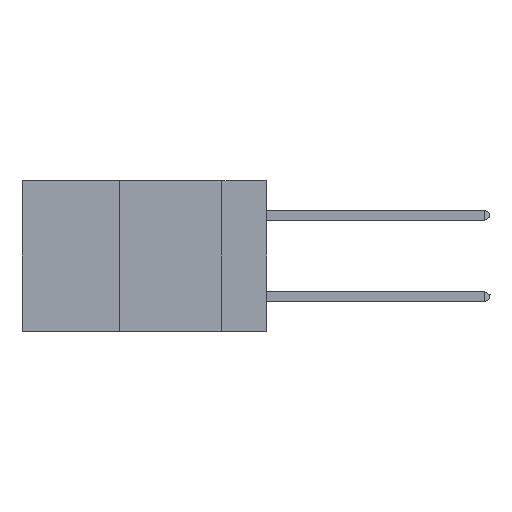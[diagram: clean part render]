
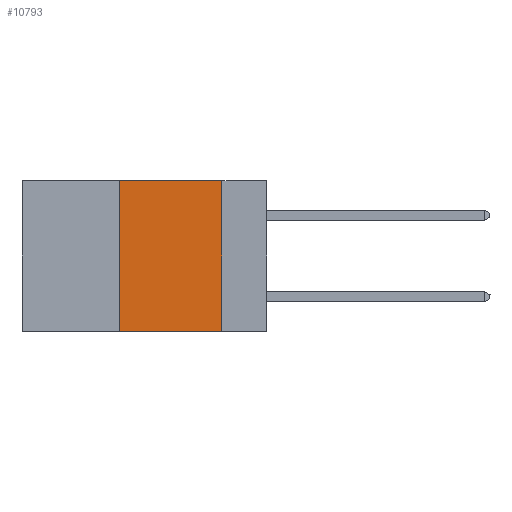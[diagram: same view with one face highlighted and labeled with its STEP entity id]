
A CAD part, left-side view. The second image highlights one B-rep face of the part: STEP entity #10793.
In plain terms, the highlighted planar face has unit normal (-1, 0, 0).
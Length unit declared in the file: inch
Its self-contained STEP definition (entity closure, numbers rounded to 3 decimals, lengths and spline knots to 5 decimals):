
#377 = CARTESIAN_POINT ( 'NONE',  ( 0., 0.6, 0. ) ) ;
#680 = VERTEX_POINT ( 'NONE', #32579 ) ;
#2504 = VECTOR ( 'NONE', #35628, 39.37008 ) ;
#5538 = EDGE_CURVE ( 'NONE', #14197, #9366, #15373, .T. ) ;
#5864 = LINE ( 'NONE', #19450, #25322 ) ;
#6317 = AXIS2_PLACEMENT_3D ( 'NONE', #377, #20652, #9364 ) ;
#6993 = LINE ( 'NONE', #20577, #8406 ) ;
#8406 = VECTOR ( 'NONE', #10543, 39.37008 ) ;
#9364 = DIRECTION ( 'NONE',  ( 0., 0., -1. ) ) ;
#9366 = VERTEX_POINT ( 'NONE', #12201 ) ;
#10543 = DIRECTION ( 'NONE',  ( 0., 0., 1. ) ) ;
#10793 = ADVANCED_FACE ( 'NONE', ( #34225 ), #23975, .F. ) ;
#11990 = EDGE_LOOP ( 'NONE', ( #38870, #13612, #29102, #24607 ) ) ;
#12201 = CARTESIAN_POINT ( 'NONE',  ( 0., 0.11, -0.37 ) ) ;
#13612 = ORIENTED_EDGE ( 'NONE', *, *, #32948, .F. ) ;
#14197 = VERTEX_POINT ( 'NONE', #16687 ) ;
#15373 = LINE ( 'NONE', #38962, #2504 ) ;
#16104 = DIRECTION ( 'NONE',  ( 0., -1., 0. ) ) ;
#16687 = CARTESIAN_POINT ( 'NONE',  ( 0., 0.11, 0. ) ) ;
#19450 = CARTESIAN_POINT ( 'NONE',  ( 0., 0.6, 0. ) ) ;
#20029 = LINE ( 'NONE', #33604, #41135 ) ;
#20577 = CARTESIAN_POINT ( 'NONE',  ( 0., 0.36, 0. ) ) ;
#20652 = DIRECTION ( 'NONE',  ( 1., 0., 0. ) ) ;
#23585 = DIRECTION ( 'NONE',  ( 0., -1., 0. ) ) ;
#23975 = PLANE ( 'NONE',  #6317 ) ;
#24607 = ORIENTED_EDGE ( 'NONE', *, *, #25086, .T. ) ;
#25086 = EDGE_CURVE ( 'NONE', #30672, #9366, #20029, .T. ) ;
#25322 = VECTOR ( 'NONE', #16104, 39.37008 ) ;
#26086 = EDGE_CURVE ( 'NONE', #30672, #680, #6993, .T. ) ;
#29102 = ORIENTED_EDGE ( 'NONE', *, *, #26086, .F. ) ;
#30672 = VERTEX_POINT ( 'NONE', #34568 ) ;
#32579 = CARTESIAN_POINT ( 'NONE',  ( 0., 0.36, 0. ) ) ;
#32948 = EDGE_CURVE ( 'NONE', #680, #14197, #5864, .T. ) ;
#33604 = CARTESIAN_POINT ( 'NONE',  ( 0., 0.6, -0.37 ) ) ;
#34225 = FACE_OUTER_BOUND ( 'NONE', #11990, .T. ) ;
#34568 = CARTESIAN_POINT ( 'NONE',  ( 0., 0.36, -0.37 ) ) ;
#35628 = DIRECTION ( 'NONE',  ( 0., 0., -1. ) ) ;
#38870 = ORIENTED_EDGE ( 'NONE', *, *, #5538, .F. ) ;
#38962 = CARTESIAN_POINT ( 'NONE',  ( 0., 0.11, 0. ) ) ;
#41135 = VECTOR ( 'NONE', #23585, 39.37008 ) ;
